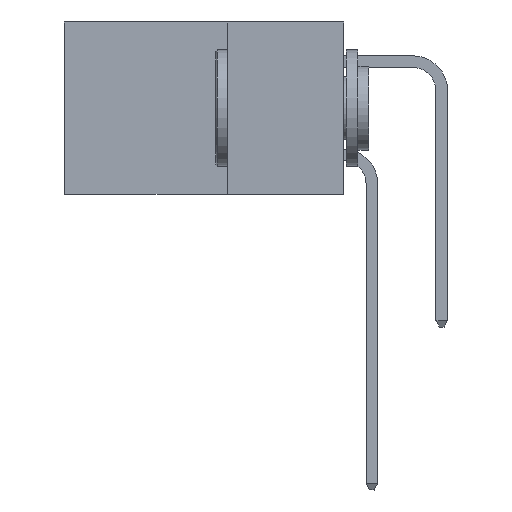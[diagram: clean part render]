
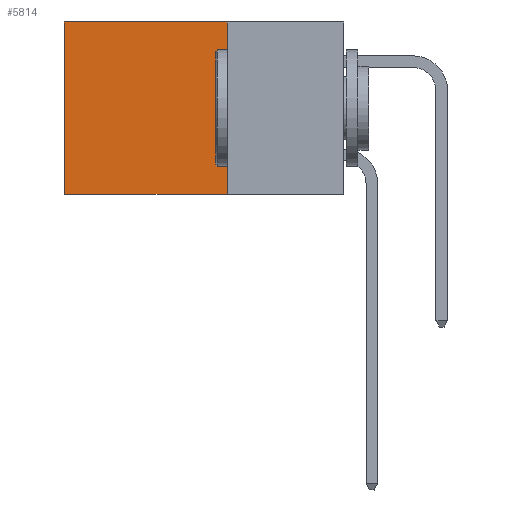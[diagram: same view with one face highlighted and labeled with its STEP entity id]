
A CAD part, left-side view. The second image highlights one B-rep face of the part: STEP entity #5814.
In plain terms, the highlighted planar face has unit normal (-1, 0, 0).
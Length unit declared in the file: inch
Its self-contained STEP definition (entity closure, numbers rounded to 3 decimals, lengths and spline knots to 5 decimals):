
#65 = DIRECTION ( 'NONE',  ( 0., 1., 0. ) ) ;
#185 = EDGE_LOOP ( 'NONE', ( #4458, #5749, #517, #10060 ) ) ;
#517 = ORIENTED_EDGE ( 'NONE', *, *, #9149, .F. ) ;
#704 = DIRECTION ( 'NONE',  ( 0., 0., -1. ) ) ;
#854 = DIRECTION ( 'NONE',  ( 0., 1., 0. ) ) ;
#1299 = LINE ( 'NONE', #3124, #7474 ) ;
#1713 = PLANE ( 'NONE',  #6883 ) ;
#1831 = VECTOR ( 'NONE', #704, 39.37008 ) ;
#1950 = EDGE_CURVE ( 'NONE', #8624, #4650, #9595, .T. ) ;
#2187 = DIRECTION ( 'NONE',  ( 0., 0., -1. ) ) ;
#2373 = EDGE_CURVE ( 'NONE', #4187, #9079, #2790, .T. ) ;
#2790 = LINE ( 'NONE', #6651, #6210 ) ;
#3124 = CARTESIAN_POINT ( 'NONE',  ( 0.2615, 0.25, -0.37 ) ) ;
#4187 = VERTEX_POINT ( 'NONE', #11449 ) ;
#4458 = ORIENTED_EDGE ( 'NONE', *, *, #5385, .T. ) ;
#4629 = CARTESIAN_POINT ( 'NONE',  ( 0.2615, 0.6, -0.37 ) ) ;
#4650 = VERTEX_POINT ( 'NONE', #11435 ) ;
#5368 = FACE_OUTER_BOUND ( 'NONE', #185, .T. ) ;
#5385 = EDGE_CURVE ( 'NONE', #9079, #4650, #12354, .T. ) ;
#5749 = ORIENTED_EDGE ( 'NONE', *, *, #1950, .F. ) ;
#5814 = ADVANCED_FACE ( 'NONE', ( #5368 ), #1713, .F. ) ;
#6210 = VECTOR ( 'NONE', #65, 39.37008 ) ;
#6324 = CARTESIAN_POINT ( 'NONE',  ( 0.2615, 0.25, -0.37 ) ) ;
#6651 = CARTESIAN_POINT ( 'NONE',  ( 0.2615, 0.25, 0. ) ) ;
#6883 = AXIS2_PLACEMENT_3D ( 'NONE', #6324, #9368, #7594 ) ;
#7474 = VECTOR ( 'NONE', #2187, 39.37008 ) ;
#7476 = CARTESIAN_POINT ( 'NONE',  ( 0.2615, 0.6, 0. ) ) ;
#7594 = DIRECTION ( 'NONE',  ( 0., 0., -1. ) ) ;
#8030 = VECTOR ( 'NONE', #854, 39.37008 ) ;
#8574 = CARTESIAN_POINT ( 'NONE',  ( 0.2615, 0.25, -0.37 ) ) ;
#8624 = VERTEX_POINT ( 'NONE', #8574 ) ;
#8830 = CARTESIAN_POINT ( 'NONE',  ( 0.2615, 0.25, -0.37 ) ) ;
#9079 = VERTEX_POINT ( 'NONE', #7476 ) ;
#9149 = EDGE_CURVE ( 'NONE', #4187, #8624, #1299, .T. ) ;
#9368 = DIRECTION ( 'NONE',  ( 1., 0., 0. ) ) ;
#9595 = LINE ( 'NONE', #8830, #8030 ) ;
#10060 = ORIENTED_EDGE ( 'NONE', *, *, #2373, .T. ) ;
#11435 = CARTESIAN_POINT ( 'NONE',  ( 0.2615, 0.6, -0.37 ) ) ;
#11449 = CARTESIAN_POINT ( 'NONE',  ( 0.2615, 0.25, 0. ) ) ;
#12354 = LINE ( 'NONE', #4629, #1831 ) ;
